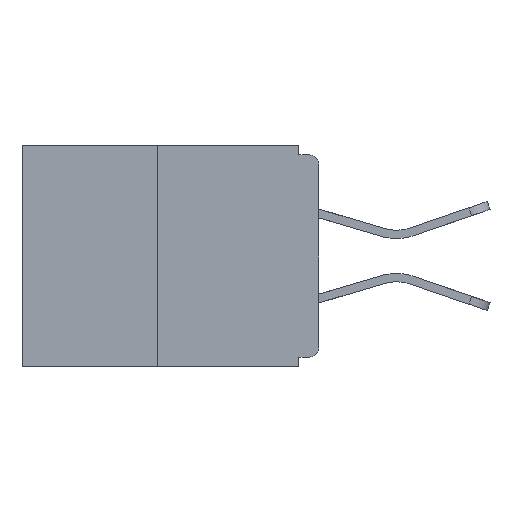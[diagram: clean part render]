
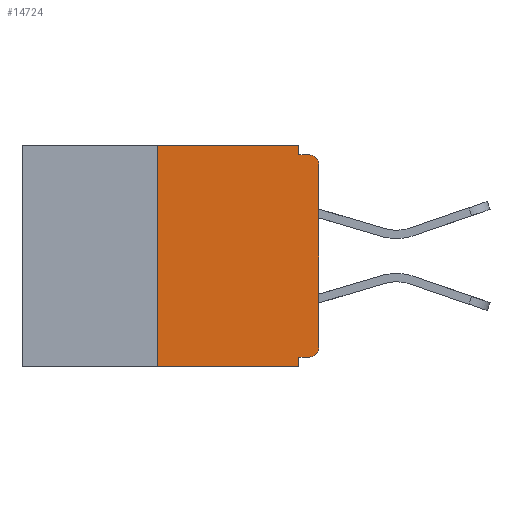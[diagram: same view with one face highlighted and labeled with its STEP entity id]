
A CAD part, left-side view. The second image highlights one B-rep face of the part: STEP entity #14724.
In plain terms, the highlighted planar face has unit normal (-1, 0, 0).
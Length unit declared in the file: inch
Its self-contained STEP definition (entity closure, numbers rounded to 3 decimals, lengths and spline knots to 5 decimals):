
#71 = LINE ( 'NONE', #23547, #7859 ) ;
#211 = DIRECTION ( 'NONE',  ( 0., 0., -1. ) ) ;
#274 = AXIS2_PLACEMENT_3D ( 'NONE', #24428, #13945, #11885 ) ;
#447 = CARTESIAN_POINT ( 'NONE',  ( 0., 0.031, -0.328 ) ) ;
#888 = LINE ( 'NONE', #12651, #23556 ) ;
#1064 = VECTOR ( 'NONE', #3585, 39.37008 ) ;
#1190 = CIRCLE ( 'NONE', #22345, 0.015 ) ;
#1786 = VERTEX_POINT ( 'NONE', #447 ) ;
#1837 = CARTESIAN_POINT ( 'NONE',  ( 0., 0.031, -0.343 ) ) ;
#2357 = ORIENTED_EDGE ( 'NONE', *, *, #4125, .F. ) ;
#2827 = DIRECTION ( 'NONE',  ( 0., 1., 0. ) ) ;
#3122 = ORIENTED_EDGE ( 'NONE', *, *, #25243, .T. ) ;
#3161 = LINE ( 'NONE', #15843, #9773 ) ;
#3197 = LINE ( 'NONE', #23773, #15352 ) ;
#3243 = ORIENTED_EDGE ( 'NONE', *, *, #22198, .F. ) ;
#3416 = EDGE_CURVE ( 'NONE', #27101, #16154, #7095, .T. ) ;
#3585 = DIRECTION ( 'NONE',  ( 0., -1., 0. ) ) ;
#3979 = ORIENTED_EDGE ( 'NONE', *, *, #18393, .F. ) ;
#4125 = EDGE_CURVE ( 'NONE', #13881, #17255, #3197, .T. ) ;
#4872 = VERTEX_POINT ( 'NONE', #16664 ) ;
#5897 = LINE ( 'NONE', #18472, #20491 ) ;
#6788 = EDGE_CURVE ( 'NONE', #27101, #18127, #3161, .T. ) ;
#6910 = VERTEX_POINT ( 'NONE', #10028 ) ;
#6949 = DIRECTION ( 'NONE',  ( 0., 0., -1. ) ) ;
#7095 = LINE ( 'NONE', #13447, #7401 ) ;
#7401 = VECTOR ( 'NONE', #7634, 39.37008 ) ;
#7450 = VERTEX_POINT ( 'NONE', #10829 ) ;
#7634 = DIRECTION ( 'NONE',  ( 0., -1., 0. ) ) ;
#7816 = DIRECTION ( 'NONE',  ( 0., 0., 1. ) ) ;
#7859 = VECTOR ( 'NONE', #211, 39.37008 ) ;
#8231 = EDGE_CURVE ( 'NONE', #6910, #4872, #21691, .T. ) ;
#9285 = ORIENTED_EDGE ( 'NONE', *, *, #26816, .T. ) ;
#9773 = VECTOR ( 'NONE', #24265, 39.37008 ) ;
#10028 = CARTESIAN_POINT ( 'NONE',  ( 0., 0., -0.03 ) ) ;
#10670 = ORIENTED_EDGE ( 'NONE', *, *, #3416, .T. ) ;
#10829 = CARTESIAN_POINT ( 'NONE',  ( 0., 0.015, -0.328 ) ) ;
#11750 = LINE ( 'NONE', #14071, #1064 ) ;
#11885 = DIRECTION ( 'NONE',  ( 0., 0., -1. ) ) ;
#12651 = CARTESIAN_POINT ( 'NONE',  ( 0., 0., -0.328 ) ) ;
#13447 = CARTESIAN_POINT ( 'NONE',  ( 0., 0.46, -0.343 ) ) ;
#13548 = DIRECTION ( 'NONE',  ( 0., 0., -1. ) ) ;
#13881 = VERTEX_POINT ( 'NONE', #19558 ) ;
#13945 = DIRECTION ( 'NONE',  ( 1., 0., 0. ) ) ;
#14071 = CARTESIAN_POINT ( 'NONE',  ( 0., 0., -0.015 ) ) ;
#14724 = ADVANCED_FACE ( 'NONE', ( #20179 ), #26523, .F. ) ;
#15211 = EDGE_CURVE ( 'NONE', #18127, #13881, #5897, .T. ) ;
#15216 = DIRECTION ( 'NONE',  ( -1., 0., 0. ) ) ;
#15352 = VECTOR ( 'NONE', #13548, 39.37008 ) ;
#15583 = EDGE_LOOP ( 'NONE', ( #16856, #20560, #10670, #3979, #16934, #9285, #3122, #18120, #3243, #2357 ) ) ;
#15843 = CARTESIAN_POINT ( 'NONE',  ( 0., 0.25, 0. ) ) ;
#16154 = VERTEX_POINT ( 'NONE', #1837 ) ;
#16664 = CARTESIAN_POINT ( 'NONE',  ( 0., 0.015, -0.015 ) ) ;
#16856 = ORIENTED_EDGE ( 'NONE', *, *, #15211, .F. ) ;
#16934 = ORIENTED_EDGE ( 'NONE', *, *, #22319, .F. ) ;
#17255 = VERTEX_POINT ( 'NONE', #24091 ) ;
#17843 = DIRECTION ( 'NONE',  ( 0., 0., -1. ) ) ;
#18120 = ORIENTED_EDGE ( 'NONE', *, *, #8231, .T. ) ;
#18127 = VERTEX_POINT ( 'NONE', #26345 ) ;
#18393 = EDGE_CURVE ( 'NONE', #1786, #16154, #71, .T. ) ;
#18472 = CARTESIAN_POINT ( 'NONE',  ( 0., 0.46, 0. ) ) ;
#18735 = DIRECTION ( 'NONE',  ( 0., -1., 0. ) ) ;
#19383 = CARTESIAN_POINT ( 'NONE',  ( 0., 0.015, -0.03 ) ) ;
#19558 = CARTESIAN_POINT ( 'NONE',  ( 0., 0.031, 0. ) ) ;
#20179 = FACE_OUTER_BOUND ( 'NONE', #15583, .T. ) ;
#20364 = AXIS2_PLACEMENT_3D ( 'NONE', #19383, #21580, #17843 ) ;
#20491 = VECTOR ( 'NONE', #18735, 39.37008 ) ;
#20560 = ORIENTED_EDGE ( 'NONE', *, *, #6788, .F. ) ;
#21395 = VECTOR ( 'NONE', #7816, 39.37008 ) ;
#21580 = DIRECTION ( 'NONE',  ( -1., 0., 0. ) ) ;
#21691 = CIRCLE ( 'NONE', #20364, 0.015 ) ;
#22198 = EDGE_CURVE ( 'NONE', #17255, #4872, #11750, .T. ) ;
#22319 = EDGE_CURVE ( 'NONE', #7450, #1786, #888, .T. ) ;
#22345 = AXIS2_PLACEMENT_3D ( 'NONE', #26012, #15216, #6949 ) ;
#22466 = CARTESIAN_POINT ( 'NONE',  ( 0., 0., -0.313 ) ) ;
#23547 = CARTESIAN_POINT ( 'NONE',  ( 0., 0.031, -0.343 ) ) ;
#23556 = VECTOR ( 'NONE', #2827, 39.37008 ) ;
#23773 = CARTESIAN_POINT ( 'NONE',  ( 0., 0.031, 0. ) ) ;
#24091 = CARTESIAN_POINT ( 'NONE',  ( 0., 0.031, -0.015 ) ) ;
#24265 = DIRECTION ( 'NONE',  ( 0., 0., 1. ) ) ;
#24428 = CARTESIAN_POINT ( 'NONE',  ( 0., 0.46, 0. ) ) ;
#24783 = CARTESIAN_POINT ( 'NONE',  ( 0., 0., 0. ) ) ;
#25057 = VERTEX_POINT ( 'NONE', #22466 ) ;
#25243 = EDGE_CURVE ( 'NONE', #25057, #6910, #26752, .T. ) ;
#25562 = CARTESIAN_POINT ( 'NONE',  ( 0., 0.25, -0.343 ) ) ;
#26012 = CARTESIAN_POINT ( 'NONE',  ( 0., 0.015, -0.313 ) ) ;
#26345 = CARTESIAN_POINT ( 'NONE',  ( 0., 0.25, 0. ) ) ;
#26523 = PLANE ( 'NONE',  #274 ) ;
#26752 = LINE ( 'NONE', #24783, #21395 ) ;
#26816 = EDGE_CURVE ( 'NONE', #7450, #25057, #1190, .T. ) ;
#27101 = VERTEX_POINT ( 'NONE', #25562 ) ;
